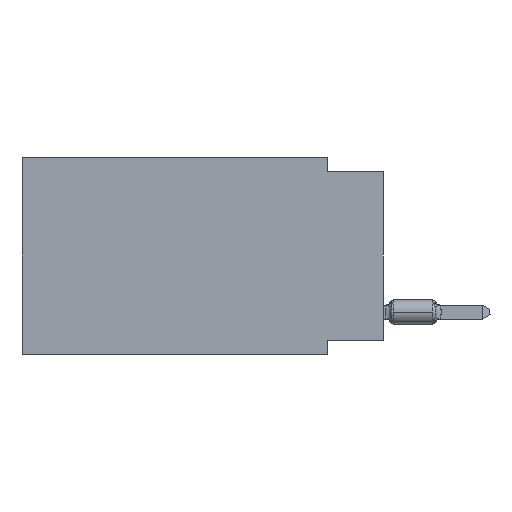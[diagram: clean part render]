
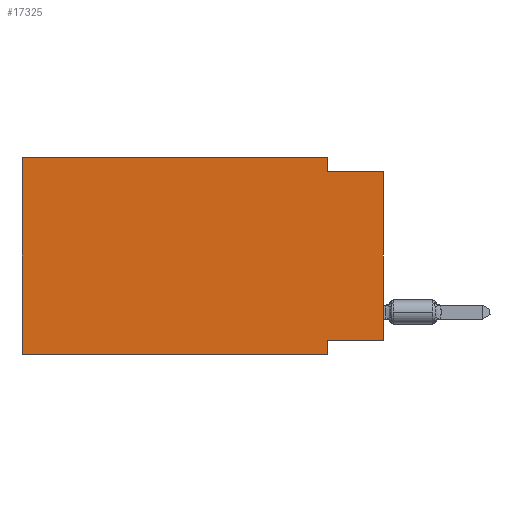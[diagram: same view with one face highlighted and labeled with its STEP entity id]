
A CAD part, left-side view. The second image highlights one B-rep face of the part: STEP entity #17325.
In plain terms, the highlighted planar face has unit normal (-1, 0, 0).
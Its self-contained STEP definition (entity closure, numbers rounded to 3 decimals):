
#218 = ORIENTED_EDGE ( 'NONE', *, *, #88714, .F. ) ;
#1896 = CARTESIAN_POINT ( 'NONE',  ( 0., 2.54, 0. ) ) ;
#3260 = CARTESIAN_POINT ( 'NONE',  ( 0., 16.383, 0. ) ) ;
#5791 = VECTOR ( 'NONE', #55679, 1000. ) ;
#12368 = CARTESIAN_POINT ( 'NONE',  ( 0., 0., -8.255 ) ) ;
#13094 = VECTOR ( 'NONE', #87807, 1000. ) ;
#15481 = CARTESIAN_POINT ( 'NONE',  ( 0., 2.54, -0.635 ) ) ;
#15546 = AXIS2_PLACEMENT_3D ( 'NONE', #3260, #80032, #18108 ) ;
#16870 = VERTEX_POINT ( 'NONE', #76744 ) ;
#17292 = CARTESIAN_POINT ( 'NONE',  ( 0., 2.54, -8.89 ) ) ;
#17325 = ADVANCED_FACE ( 'NONE', ( #79516 ), #57496, .F. ) ;
#17572 = CARTESIAN_POINT ( 'NONE',  ( 0., 16.383, -8.89 ) ) ;
#17599 = VERTEX_POINT ( 'NONE', #47180 ) ;
#18075 = LINE ( 'NONE', #17572, #51627 ) ;
#18108 = DIRECTION ( 'NONE',  ( 0., 0., -1. ) ) ;
#19301 = CARTESIAN_POINT ( 'NONE',  ( 0., 0., -0.635 ) ) ;
#22849 = VECTOR ( 'NONE', #30722, 1000. ) ;
#23203 = EDGE_CURVE ( 'NONE', #36339, #52716, #26416, .T. ) ;
#23643 = DIRECTION ( 'NONE',  ( 0., -1., 0. ) ) ;
#26416 = LINE ( 'NONE', #80647, #13094 ) ;
#27383 = EDGE_CURVE ( 'NONE', #52716, #71758, #32835, .T. ) ;
#30539 = ORIENTED_EDGE ( 'NONE', *, *, #71235, .F. ) ;
#30722 = DIRECTION ( 'NONE',  ( 0., 0., -1. ) ) ;
#31922 = CARTESIAN_POINT ( 'NONE',  ( 0., 0., -0.635 ) ) ;
#32337 = EDGE_CURVE ( 'NONE', #17599, #86298, #56059, .T. ) ;
#32835 = LINE ( 'NONE', #62544, #87072 ) ;
#33606 = LINE ( 'NONE', #1896, #22849 ) ;
#34892 = LINE ( 'NONE', #12368, #69187 ) ;
#36339 = VERTEX_POINT ( 'NONE', #52819 ) ;
#37748 = VERTEX_POINT ( 'NONE', #15481 ) ;
#38498 = VERTEX_POINT ( 'NONE', #63688 ) ;
#43575 = DIRECTION ( 'NONE',  ( 0., 1., 0. ) ) ;
#45989 = CARTESIAN_POINT ( 'NONE',  ( 0., 0., 0. ) ) ;
#46481 = LINE ( 'NONE', #17292, #5791 ) ;
#47180 = CARTESIAN_POINT ( 'NONE',  ( 0., 0., -8.255 ) ) ;
#49804 = EDGE_CURVE ( 'NONE', #36339, #16870, #18075, .T. ) ;
#50097 = ORIENTED_EDGE ( 'NONE', *, *, #32337, .T. ) ;
#51627 = VECTOR ( 'NONE', #63118, 1000. ) ;
#52716 = VERTEX_POINT ( 'NONE', #86498 ) ;
#52819 = CARTESIAN_POINT ( 'NONE',  ( 0., 16.383, -8.89 ) ) ;
#55679 = DIRECTION ( 'NONE',  ( 0., 0., -1. ) ) ;
#56059 = LINE ( 'NONE', #45989, #59958 ) ;
#56558 = DIRECTION ( 'NONE',  ( 0., 0., 1. ) ) ;
#57496 = PLANE ( 'NONE',  #15546 ) ;
#59055 = EDGE_LOOP ( 'NONE', ( #50097, #85137, #30539, #71514, #63571, #60434, #61626, #218 ) ) ;
#59958 = VECTOR ( 'NONE', #56558, 1000. ) ;
#60434 = ORIENTED_EDGE ( 'NONE', *, *, #49804, .T. ) ;
#61626 = ORIENTED_EDGE ( 'NONE', *, *, #96777, .F. ) ;
#62544 = CARTESIAN_POINT ( 'NONE',  ( 0., 16.383, 0. ) ) ;
#63118 = DIRECTION ( 'NONE',  ( 0., -1., 0. ) ) ;
#63571 = ORIENTED_EDGE ( 'NONE', *, *, #23203, .F. ) ;
#63688 = CARTESIAN_POINT ( 'NONE',  ( 0., 2.54, -8.255 ) ) ;
#69187 = VECTOR ( 'NONE', #43575, 1000. ) ;
#71235 = EDGE_CURVE ( 'NONE', #71758, #37748, #33606, .T. ) ;
#71514 = ORIENTED_EDGE ( 'NONE', *, *, #27383, .F. ) ;
#71758 = VERTEX_POINT ( 'NONE', #74374 ) ;
#72978 = EDGE_CURVE ( 'NONE', #37748, #86298, #87867, .T. ) ;
#74374 = CARTESIAN_POINT ( 'NONE',  ( 0., 2.54, 0. ) ) ;
#76744 = CARTESIAN_POINT ( 'NONE',  ( 0., 2.54, -8.89 ) ) ;
#79516 = FACE_OUTER_BOUND ( 'NONE', #59055, .T. ) ;
#80032 = DIRECTION ( 'NONE',  ( 1., 0., 0. ) ) ;
#80210 = DIRECTION ( 'NONE',  ( 0., -1., 0. ) ) ;
#80647 = CARTESIAN_POINT ( 'NONE',  ( 0., 16.383, 0. ) ) ;
#85005 = VECTOR ( 'NONE', #80210, 1000. ) ;
#85137 = ORIENTED_EDGE ( 'NONE', *, *, #72978, .F. ) ;
#86298 = VERTEX_POINT ( 'NONE', #31922 ) ;
#86498 = CARTESIAN_POINT ( 'NONE',  ( 0., 16.383, 0. ) ) ;
#87072 = VECTOR ( 'NONE', #23643, 1000. ) ;
#87807 = DIRECTION ( 'NONE',  ( 0., 0., 1. ) ) ;
#87867 = LINE ( 'NONE', #19301, #85005 ) ;
#88714 = EDGE_CURVE ( 'NONE', #17599, #38498, #34892, .T. ) ;
#96777 = EDGE_CURVE ( 'NONE', #38498, #16870, #46481, .T. ) ;
